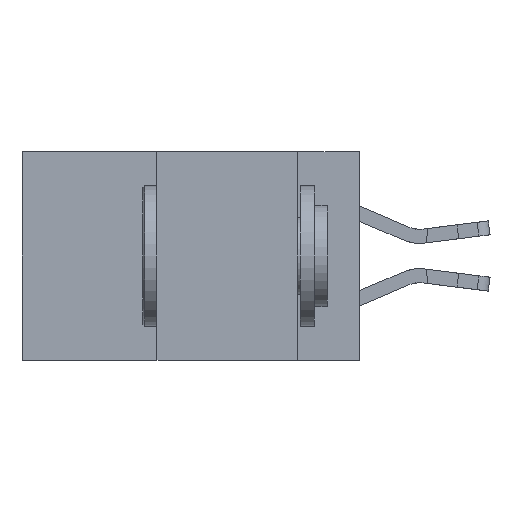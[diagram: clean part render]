
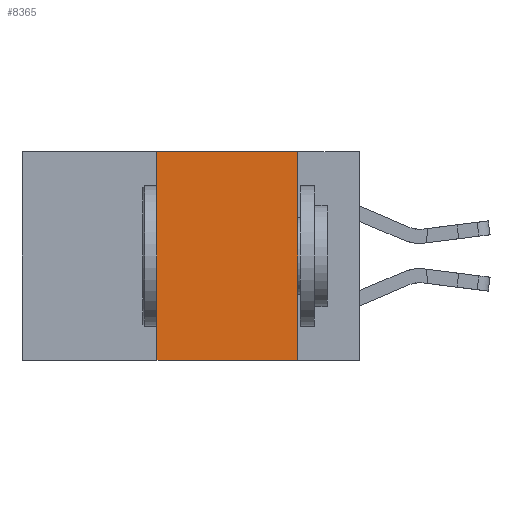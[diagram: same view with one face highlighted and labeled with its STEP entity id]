
A CAD part, left-side view. The second image highlights one B-rep face of the part: STEP entity #8365.
In plain terms, the highlighted planar face has unit normal (-1, 0, 0).
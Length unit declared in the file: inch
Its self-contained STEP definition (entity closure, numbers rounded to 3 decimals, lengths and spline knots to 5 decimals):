
#196 = VECTOR ( 'NONE', #18114, 39.37008 ) ;
#234 = EDGE_CURVE ( 'NONE', #14486, #11947, #3378, .T. ) ;
#2047 = CARTESIAN_POINT ( 'NONE',  ( 0., 0.6, 0. ) ) ;
#2664 = LINE ( 'NONE', #24372, #196 ) ;
#3378 = LINE ( 'NONE', #11366, #21965 ) ;
#3460 = CARTESIAN_POINT ( 'NONE',  ( 0., 0.11, 0. ) ) ;
#4013 = DIRECTION ( 'NONE',  ( 1., 0., 0. ) ) ;
#4132 = EDGE_CURVE ( 'NONE', #11947, #15789, #20895, .T. ) ;
#4478 = CARTESIAN_POINT ( 'NONE',  ( 0., 0.36, 0. ) ) ;
#5736 = ORIENTED_EDGE ( 'NONE', *, *, #4132, .F. ) ;
#7121 = FACE_OUTER_BOUND ( 'NONE', #14121, .T. ) ;
#7147 = CARTESIAN_POINT ( 'NONE',  ( 0., 0.11, 0. ) ) ;
#8365 = ADVANCED_FACE ( 'NONE', ( #7121 ), #13878, .F. ) ;
#8691 = LINE ( 'NONE', #3460, #18595 ) ;
#10194 = CARTESIAN_POINT ( 'NONE',  ( 0., 0.36, -0.37 ) ) ;
#10245 = EDGE_CURVE ( 'NONE', #14486, #20656, #2664, .T. ) ;
#11042 = CARTESIAN_POINT ( 'NONE',  ( 0., 0.11, -0.37 ) ) ;
#11366 = CARTESIAN_POINT ( 'NONE',  ( 0., 0.36, 0. ) ) ;
#11947 = VERTEX_POINT ( 'NONE', #4478 ) ;
#12968 = CARTESIAN_POINT ( 'NONE',  ( 0., 0.6, 0. ) ) ;
#13253 = EDGE_CURVE ( 'NONE', #15789, #20656, #8691, .T. ) ;
#13878 = PLANE ( 'NONE',  #21089 ) ;
#14121 = EDGE_LOOP ( 'NONE', ( #18579, #5736, #19303, #24884 ) ) ;
#14486 = VERTEX_POINT ( 'NONE', #10194 ) ;
#15789 = VERTEX_POINT ( 'NONE', #7147 ) ;
#16860 = VECTOR ( 'NONE', #22794, 39.37008 ) ;
#17649 = DIRECTION ( 'NONE',  ( 0., 0., -1. ) ) ;
#17879 = DIRECTION ( 'NONE',  ( 0., 0., -1. ) ) ;
#18114 = DIRECTION ( 'NONE',  ( 0., -1., 0. ) ) ;
#18579 = ORIENTED_EDGE ( 'NONE', *, *, #13253, .F. ) ;
#18595 = VECTOR ( 'NONE', #17649, 39.37008 ) ;
#19303 = ORIENTED_EDGE ( 'NONE', *, *, #234, .F. ) ;
#20656 = VERTEX_POINT ( 'NONE', #11042 ) ;
#20895 = LINE ( 'NONE', #12968, #16860 ) ;
#21089 = AXIS2_PLACEMENT_3D ( 'NONE', #2047, #4013, #17879 ) ;
#21965 = VECTOR ( 'NONE', #23164, 39.37008 ) ;
#22794 = DIRECTION ( 'NONE',  ( 0., -1., 0. ) ) ;
#23164 = DIRECTION ( 'NONE',  ( 0., 0., 1. ) ) ;
#24372 = CARTESIAN_POINT ( 'NONE',  ( 0., 0.6, -0.37 ) ) ;
#24884 = ORIENTED_EDGE ( 'NONE', *, *, #10245, .T. ) ;
